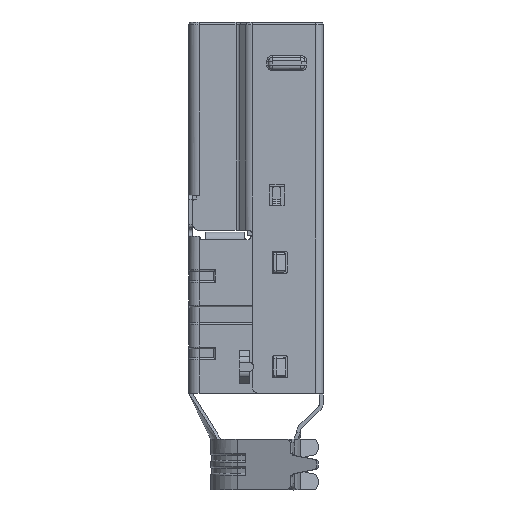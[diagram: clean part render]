
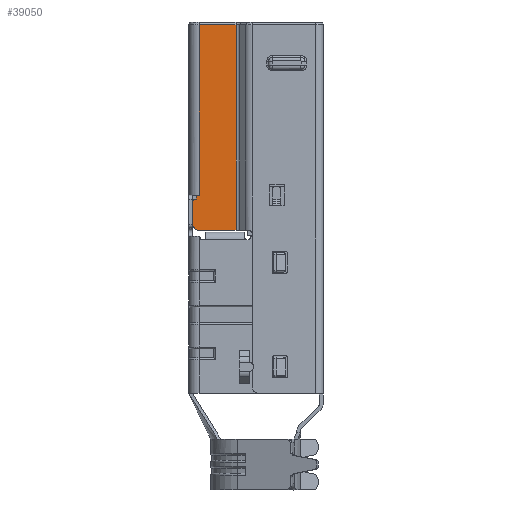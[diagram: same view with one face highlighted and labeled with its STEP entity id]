
A CAD part, left-side view. The second image highlights one B-rep face of the part: STEP entity #39050.
In plain terms, the highlighted planar face has unit normal (-1, 0, 0).
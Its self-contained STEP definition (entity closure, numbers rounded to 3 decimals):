
#484 = EDGE_CURVE ( 'NONE', #35190, #19256, #1002, .T. ) ;
#510 = EDGE_CURVE ( 'NONE', #9733, #19256, #20271, .T. ) ;
#834 = EDGE_CURVE ( 'NONE', #5498, #9733, #26271, .T. ) ;
#1002 = LINE ( 'NONE', #39321, #31634 ) ;
#1891 = DIRECTION ( 'NONE',  ( 0., 1., 0. ) ) ;
#2979 = CARTESIAN_POINT ( 'NONE',  ( -3.196, 4.825, -13.45 ) ) ;
#3558 = DIRECTION ( 'NONE',  ( 0., 0., -1. ) ) ;
#4008 = AXIS2_PLACEMENT_3D ( 'NONE', #31660, #35435, #43166 ) ;
#4305 = CARTESIAN_POINT ( 'NONE',  ( -3.196, 6.209, -13.75 ) ) ;
#5498 = VERTEX_POINT ( 'NONE', #46019 ) ;
#6387 = CARTESIAN_POINT ( 'NONE',  ( -3.196, 3.073, -16.469 ) ) ;
#7264 = EDGE_CURVE ( 'NONE', #46837, #16512, #49340, .T. ) ;
#8086 = ORIENTED_EDGE ( 'NONE', *, *, #484, .T. ) ;
#8704 = EDGE_CURVE ( 'NONE', #16512, #26098, #14767, .T. ) ;
#9147 = DIRECTION ( 'NONE',  ( 1., 0., 0. ) ) ;
#9227 = ORIENTED_EDGE ( 'NONE', *, *, #10326, .T. ) ;
#9733 = VERTEX_POINT ( 'NONE', #28064 ) ;
#9850 = ORIENTED_EDGE ( 'NONE', *, *, #7264, .T. ) ;
#9873 = PLANE ( 'NONE',  #45419 ) ;
#10326 = EDGE_CURVE ( 'NONE', #26098, #16686, #35213, .T. ) ;
#11527 = CARTESIAN_POINT ( 'NONE',  ( -3.196, 6.309, -13.75 ) ) ;
#11740 = DIRECTION ( 'NONE',  ( 0., 0., -1. ) ) ;
#12518 = CARTESIAN_POINT ( 'NONE',  ( -3.196, 3.14, -8.175 ) ) ;
#14619 = CARTESIAN_POINT ( 'NONE',  ( -3.196, 6.509, -15.65 ) ) ;
#14767 = LINE ( 'NONE', #34079, #46130 ) ;
#14968 = DIRECTION ( 'NONE',  ( 0., -1., 0. ) ) ;
#15048 = DIRECTION ( 'NONE',  ( -1., 0., 0. ) ) ;
#15822 = VECTOR ( 'NONE', #15978, 1000. ) ;
#15978 = DIRECTION ( 'NONE',  ( 0., 1., 0. ) ) ;
#16512 = VERTEX_POINT ( 'NONE', #48258 ) ;
#16686 = VERTEX_POINT ( 'NONE', #30722 ) ;
#17674 = EDGE_CURVE ( 'NONE', #22074, #5498, #43791, .T. ) ;
#18062 = ORIENTED_EDGE ( 'NONE', *, *, #23688, .F. ) ;
#18418 = CARTESIAN_POINT ( 'NONE',  ( -3.196, 6.009, -0.2 ) ) ;
#18635 = CARTESIAN_POINT ( 'NONE',  ( -3.196, 3.14, -16.15 ) ) ;
#19256 = VERTEX_POINT ( 'NONE', #18418 ) ;
#19656 = ORIENTED_EDGE ( 'NONE', *, *, #17674, .F. ) ;
#20271 = LINE ( 'NONE', #35585, #22539 ) ;
#20989 = DIRECTION ( 'NONE',  ( 0., 0., 1. ) ) ;
#22074 = VERTEX_POINT ( 'NONE', #4305 ) ;
#22539 = VECTOR ( 'NONE', #47090, 1000. ) ;
#22854 = CARTESIAN_POINT ( 'NONE',  ( -3.196, 6.209, -13.6 ) ) ;
#23028 = LINE ( 'NONE', #42298, #15822 ) ;
#23119 = DIRECTION ( 'NONE',  ( 0., -1., 0. ) ) ;
#23564 = DIRECTION ( 'NONE',  ( 0., 0., -1. ) ) ;
#23688 = EDGE_CURVE ( 'NONE', #46837, #22074, #42149, .T. ) ;
#24034 = DIRECTION ( 'NONE',  ( 0., 1., 0. ) ) ;
#24686 = VECTOR ( 'NONE', #23564, 1000. ) ;
#26098 = VERTEX_POINT ( 'NONE', #14619 ) ;
#26271 = LINE ( 'NONE', #2979, #34270 ) ;
#27285 = ORIENTED_EDGE ( 'NONE', *, *, #8704, .T. ) ;
#28064 = CARTESIAN_POINT ( 'NONE',  ( -3.196, 6.009, -13.45 ) ) ;
#29258 = ORIENTED_EDGE ( 'NONE', *, *, #834, .F. ) ;
#29711 = ORIENTED_EDGE ( 'NONE', *, *, #510, .F. ) ;
#30722 = CARTESIAN_POINT ( 'NONE',  ( -3.196, 6.009, -16.15 ) ) ;
#31634 = VECTOR ( 'NONE', #24034, 1000. ) ;
#31660 = CARTESIAN_POINT ( 'NONE',  ( -3.196, 6.009, -15.65 ) ) ;
#32276 = EDGE_CURVE ( 'NONE', #35190, #41705, #39830, .T. ) ;
#32661 = CARTESIAN_POINT ( 'NONE',  ( -3.196, 3.14, -0.2 ) ) ;
#34079 = CARTESIAN_POINT ( 'NONE',  ( -3.196, 6.509, -14.8 ) ) ;
#34270 = VECTOR ( 'NONE', #14968, 1000. ) ;
#34337 = EDGE_LOOP ( 'NONE', ( #47881, #8086, #29711, #29258, #19656, #18062, #9850, #27285, #9227, #44985 ) ) ;
#34620 = CARTESIAN_POINT ( 'NONE',  ( -3.196, 6.309, -13.95 ) ) ;
#34936 = AXIS2_PLACEMENT_3D ( 'NONE', #34620, #15048, #3558 ) ;
#35190 = VERTEX_POINT ( 'NONE', #32661 ) ;
#35213 = CIRCLE ( 'NONE', #4008, 0.5 ) ;
#35435 = DIRECTION ( 'NONE',  ( -1., 0., 0. ) ) ;
#35585 = CARTESIAN_POINT ( 'NONE',  ( -3.196, 6.009, -8.175 ) ) ;
#36214 = FACE_OUTER_BOUND ( 'NONE', #34337, .T. ) ;
#38662 = VECTOR ( 'NONE', #23119, 1000. ) ;
#39050 = ADVANCED_FACE ( 'NONE', ( #36214 ), #9873, .F. ) ;
#39321 = CARTESIAN_POINT ( 'NONE',  ( -3.196, 4.575, -0.2 ) ) ;
#39830 = LINE ( 'NONE', #12518, #24686 ) ;
#41705 = VERTEX_POINT ( 'NONE', #18635 ) ;
#42149 = LINE ( 'NONE', #46177, #38662 ) ;
#42298 = CARTESIAN_POINT ( 'NONE',  ( -3.196, 4.825, -16.15 ) ) ;
#42517 = EDGE_CURVE ( 'NONE', #41705, #16686, #23028, .T. ) ;
#42643 = VECTOR ( 'NONE', #20989, 1000. ) ;
#43166 = DIRECTION ( 'NONE',  ( 0., 0., -1. ) ) ;
#43791 = LINE ( 'NONE', #22854, #42643 ) ;
#44985 = ORIENTED_EDGE ( 'NONE', *, *, #42517, .F. ) ;
#45419 = AXIS2_PLACEMENT_3D ( 'NONE', #6387, #9147, #1891 ) ;
#46019 = CARTESIAN_POINT ( 'NONE',  ( -3.196, 6.209, -13.45 ) ) ;
#46130 = VECTOR ( 'NONE', #11740, 1000. ) ;
#46177 = CARTESIAN_POINT ( 'NONE',  ( -3.196, 6.259, -13.75 ) ) ;
#46837 = VERTEX_POINT ( 'NONE', #11527 ) ;
#47090 = DIRECTION ( 'NONE',  ( 0., 0., 1. ) ) ;
#47881 = ORIENTED_EDGE ( 'NONE', *, *, #32276, .F. ) ;
#48258 = CARTESIAN_POINT ( 'NONE',  ( -3.196, 6.509, -13.95 ) ) ;
#49340 = CIRCLE ( 'NONE', #34936, 0.2 ) ;
